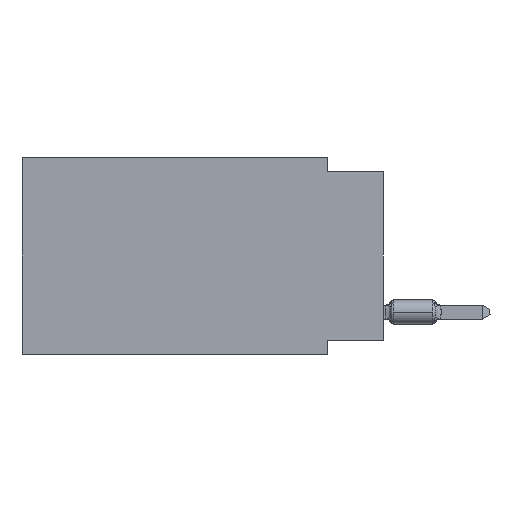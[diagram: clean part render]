
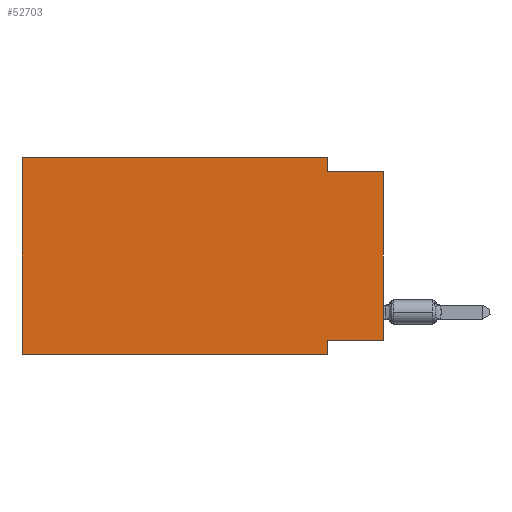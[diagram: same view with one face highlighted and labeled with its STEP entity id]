
A CAD part, left-side view. The second image highlights one B-rep face of the part: STEP entity #52703.
In plain terms, the highlighted planar face has unit normal (-1, 0, 0).
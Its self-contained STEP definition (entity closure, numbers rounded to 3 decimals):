
#800 = VECTOR ( 'NONE', #82701, 1000. ) ;
#2134 = VERTEX_POINT ( 'NONE', #19316 ) ;
#2706 = DIRECTION ( 'NONE',  ( 0., -1., 0. ) ) ;
#2783 = VECTOR ( 'NONE', #80087, 1000. ) ;
#3963 = ORIENTED_EDGE ( 'NONE', *, *, #101942, .T. ) ;
#5742 = CARTESIAN_POINT ( 'NONE',  ( 0., 2.54, -8.89 ) ) ;
#8151 = PLANE ( 'NONE',  #96133 ) ;
#11114 = CARTESIAN_POINT ( 'NONE',  ( 0., 2.54, -8.89 ) ) ;
#13209 = DIRECTION ( 'NONE',  ( 0., 0., 1. ) ) ;
#14035 = ORIENTED_EDGE ( 'NONE', *, *, #54110, .F. ) ;
#14875 = EDGE_LOOP ( 'NONE', ( #75045, #14035, #41970, #88673, #47529, #3963, #18381, #93146 ) ) ;
#16830 = DIRECTION ( 'NONE',  ( 1., 0., 0. ) ) ;
#17981 = LINE ( 'NONE', #67353, #35594 ) ;
#18381 = ORIENTED_EDGE ( 'NONE', *, *, #18725, .F. ) ;
#18725 = EDGE_CURVE ( 'NONE', #51879, #51578, #76771, .T. ) ;
#19316 = CARTESIAN_POINT ( 'NONE',  ( 0., 16.383, -8.89 ) ) ;
#20515 = VECTOR ( 'NONE', #51831, 1000. ) ;
#20808 = EDGE_CURVE ( 'NONE', #83441, #78741, #68095, .T. ) ;
#21871 = DIRECTION ( 'NONE',  ( 0., 0., 1. ) ) ;
#25494 = DIRECTION ( 'NONE',  ( 0., 0., -1. ) ) ;
#32679 = DIRECTION ( 'NONE',  ( 0., -1., 0. ) ) ;
#35594 = VECTOR ( 'NONE', #32679, 1000. ) ;
#38165 = LINE ( 'NONE', #38686, #60065 ) ;
#38686 = CARTESIAN_POINT ( 'NONE',  ( 0., 0., 0. ) ) ;
#39877 = VERTEX_POINT ( 'NONE', #84835 ) ;
#41970 = ORIENTED_EDGE ( 'NONE', *, *, #106112, .F. ) ;
#42370 = VERTEX_POINT ( 'NONE', #92607 ) ;
#47014 = LINE ( 'NONE', #63819, #2783 ) ;
#47521 = CARTESIAN_POINT ( 'NONE',  ( 0., 0., -0.635 ) ) ;
#47529 = ORIENTED_EDGE ( 'NONE', *, *, #77699, .F. ) ;
#49638 = CARTESIAN_POINT ( 'NONE',  ( 0., 0., -8.255 ) ) ;
#50460 = FACE_OUTER_BOUND ( 'NONE', #14875, .T. ) ;
#51578 = VERTEX_POINT ( 'NONE', #5742 ) ;
#51831 = DIRECTION ( 'NONE',  ( 0., -1., 0. ) ) ;
#51838 = DIRECTION ( 'NONE',  ( 0., 0., -1. ) ) ;
#51879 = VERTEX_POINT ( 'NONE', #67504 ) ;
#52703 = ADVANCED_FACE ( 'NONE', ( #50460 ), #8151, .F. ) ;
#54110 = EDGE_CURVE ( 'NONE', #42370, #104885, #69917, .T. ) ;
#54977 = LINE ( 'NONE', #77257, #72773 ) ;
#58973 = CARTESIAN_POINT ( 'NONE',  ( 0., 2.54, 0. ) ) ;
#60065 = VECTOR ( 'NONE', #21871, 1000. ) ;
#61491 = VECTOR ( 'NONE', #51838, 1000. ) ;
#63819 = CARTESIAN_POINT ( 'NONE',  ( 0., 2.54, 0. ) ) ;
#66426 = LINE ( 'NONE', #49638, #800 ) ;
#67353 = CARTESIAN_POINT ( 'NONE',  ( 0., 16.383, -8.89 ) ) ;
#67504 = CARTESIAN_POINT ( 'NONE',  ( 0., 2.54, -8.255 ) ) ;
#68095 = LINE ( 'NONE', #92480, #20515 ) ;
#68461 = EDGE_CURVE ( 'NONE', #39877, #51879, #66426, .T. ) ;
#69917 = LINE ( 'NONE', #95912, #71836 ) ;
#71836 = VECTOR ( 'NONE', #2706, 1000. ) ;
#72773 = VECTOR ( 'NONE', #13209, 1000. ) ;
#74331 = CARTESIAN_POINT ( 'NONE',  ( 0., 16.383, 0. ) ) ;
#75045 = ORIENTED_EDGE ( 'NONE', *, *, #86531, .T. ) ;
#76771 = LINE ( 'NONE', #11114, #61491 ) ;
#77257 = CARTESIAN_POINT ( 'NONE',  ( 0., 16.383, 0. ) ) ;
#77699 = EDGE_CURVE ( 'NONE', #2134, #83441, #54977, .T. ) ;
#78741 = VERTEX_POINT ( 'NONE', #58973 ) ;
#80087 = DIRECTION ( 'NONE',  ( 0., 0., -1. ) ) ;
#82701 = DIRECTION ( 'NONE',  ( 0., 1., 0. ) ) ;
#83441 = VERTEX_POINT ( 'NONE', #101505 ) ;
#84835 = CARTESIAN_POINT ( 'NONE',  ( 0., 0., -8.255 ) ) ;
#86531 = EDGE_CURVE ( 'NONE', #39877, #104885, #38165, .T. ) ;
#88673 = ORIENTED_EDGE ( 'NONE', *, *, #20808, .F. ) ;
#92480 = CARTESIAN_POINT ( 'NONE',  ( 0., 16.383, 0. ) ) ;
#92607 = CARTESIAN_POINT ( 'NONE',  ( 0., 2.54, -0.635 ) ) ;
#93146 = ORIENTED_EDGE ( 'NONE', *, *, #68461, .F. ) ;
#95912 = CARTESIAN_POINT ( 'NONE',  ( 0., 0., -0.635 ) ) ;
#96133 = AXIS2_PLACEMENT_3D ( 'NONE', #74331, #16830, #25494 ) ;
#101505 = CARTESIAN_POINT ( 'NONE',  ( 0., 16.383, 0. ) ) ;
#101942 = EDGE_CURVE ( 'NONE', #2134, #51578, #17981, .T. ) ;
#104885 = VERTEX_POINT ( 'NONE', #47521 ) ;
#106112 = EDGE_CURVE ( 'NONE', #78741, #42370, #47014, .T. ) ;
